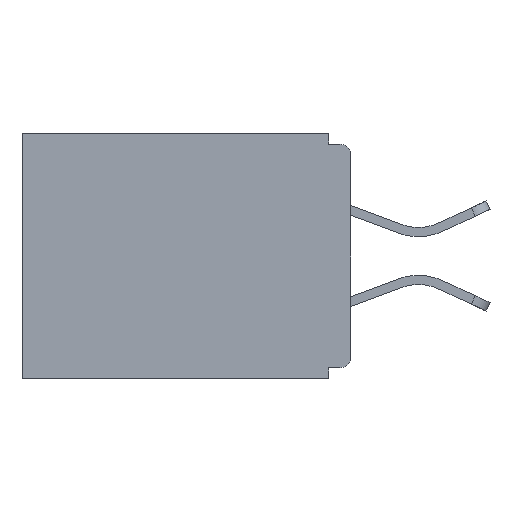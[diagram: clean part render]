
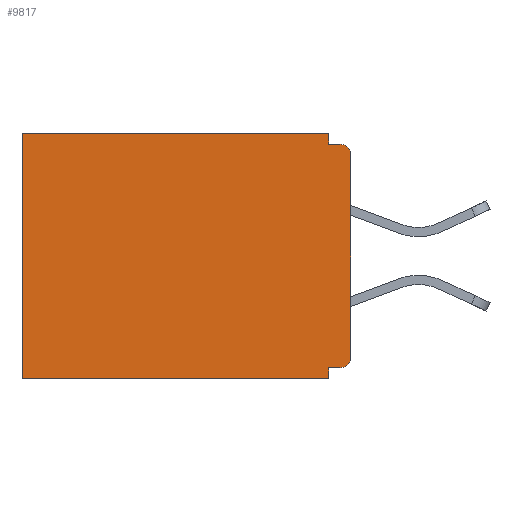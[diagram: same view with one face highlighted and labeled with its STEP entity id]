
A CAD part, left-side view. The second image highlights one B-rep face of the part: STEP entity #9817.
In plain terms, the highlighted planar face has unit normal (-1, 0, 0).
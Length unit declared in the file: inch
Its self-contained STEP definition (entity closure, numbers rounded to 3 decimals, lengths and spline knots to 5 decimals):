
#53 = VERTEX_POINT ( 'NONE', #4305 ) ;
#56 = DIRECTION ( 'NONE',  ( 0., 0., -1. ) ) ;
#120 = VECTOR ( 'NONE', #7833, 39.37008 ) ;
#472 = LINE ( 'NONE', #9594, #2384 ) ;
#532 = ORIENTED_EDGE ( 'NONE', *, *, #11973, .T. ) ;
#645 = DIRECTION ( 'NONE',  ( 0., 0., -1. ) ) ;
#818 = ORIENTED_EDGE ( 'NONE', *, *, #10296, .F. ) ;
#843 = EDGE_CURVE ( 'NONE', #11170, #13612, #1745, .T. ) ;
#1745 = LINE ( 'NONE', #5186, #12698 ) ;
#2384 = VECTOR ( 'NONE', #6439, 39.37008 ) ;
#2605 = DIRECTION ( 'NONE',  ( 0., 0., -1. ) ) ;
#2826 = CARTESIAN_POINT ( 'NONE',  ( 0.298, 0., -0.015 ) ) ;
#2828 = CARTESIAN_POINT ( 'NONE',  ( 0.298, 0.46, 0. ) ) ;
#2873 = DIRECTION ( 'NONE',  ( 0., -1., 0. ) ) ;
#2877 = LINE ( 'NONE', #7743, #120 ) ;
#2940 = LINE ( 'NONE', #10878, #8274 ) ;
#3093 = CARTESIAN_POINT ( 'NONE',  ( 0.298, 0., 0. ) ) ;
#3096 = EDGE_CURVE ( 'NONE', #9137, #13612, #11832, .T. ) ;
#3259 = DIRECTION ( 'NONE',  ( 0., 1., 0. ) ) ;
#3328 = DIRECTION ( 'NONE',  ( 0., 0., -1. ) ) ;
#3933 = LINE ( 'NONE', #2826, #5913 ) ;
#4124 = EDGE_CURVE ( 'NONE', #4360, #11170, #4340, .T. ) ;
#4277 = VERTEX_POINT ( 'NONE', #7335 ) ;
#4305 = CARTESIAN_POINT ( 'NONE',  ( 0.298, 0.015, -0.328 ) ) ;
#4340 = LINE ( 'NONE', #5867, #11533 ) ;
#4360 = VERTEX_POINT ( 'NONE', #8013 ) ;
#4390 = DIRECTION ( 'NONE',  ( 0., 0., -1. ) ) ;
#4479 = VECTOR ( 'NONE', #4390, 39.37008 ) ;
#4544 = CARTESIAN_POINT ( 'NONE',  ( 0.298, 0.031, 0. ) ) ;
#4630 = DIRECTION ( 'NONE',  ( -1., 0., 0. ) ) ;
#4906 = ORIENTED_EDGE ( 'NONE', *, *, #8773, .T. ) ;
#5059 = VERTEX_POINT ( 'NONE', #4544 ) ;
#5186 = CARTESIAN_POINT ( 'NONE',  ( 0.298, 0., -0.343 ) ) ;
#5240 = CARTESIAN_POINT ( 'NONE',  ( 0.298, 0.46, -0.343 ) ) ;
#5397 = ORIENTED_EDGE ( 'NONE', *, *, #10454, .T. ) ;
#5398 = DIRECTION ( 'NONE',  ( 1., 0., 0. ) ) ;
#5611 = EDGE_CURVE ( 'NONE', #11271, #8356, #2940, .T. ) ;
#5690 = CIRCLE ( 'NONE', #11031, 0.015 ) ;
#5867 = CARTESIAN_POINT ( 'NONE',  ( 0.298, 0.031, -0.343 ) ) ;
#5870 = DIRECTION ( 'NONE',  ( -1., 0., 0. ) ) ;
#5886 = ORIENTED_EDGE ( 'NONE', *, *, #12929, .F. ) ;
#5913 = VECTOR ( 'NONE', #2873, 39.37008 ) ;
#6171 = AXIS2_PLACEMENT_3D ( 'NONE', #3093, #5398, #56 ) ;
#6225 = CARTESIAN_POINT ( 'NONE',  ( 0.298, 0., -0.313 ) ) ;
#6432 = ORIENTED_EDGE ( 'NONE', *, *, #843, .F. ) ;
#6437 = CARTESIAN_POINT ( 'NONE',  ( 0.298, 0., -0.328 ) ) ;
#6439 = DIRECTION ( 'NONE',  ( 0., 1., 0. ) ) ;
#6514 = CARTESIAN_POINT ( 'NONE',  ( 0.298, 0.46, 0. ) ) ;
#6520 = ORIENTED_EDGE ( 'NONE', *, *, #4124, .F. ) ;
#6580 = DIRECTION ( 'NONE',  ( 0., 0., -1. ) ) ;
#7241 = DIRECTION ( 'NONE',  ( 0., 1., 0. ) ) ;
#7335 = CARTESIAN_POINT ( 'NONE',  ( 0.298, 0.015, -0.015 ) ) ;
#7743 = CARTESIAN_POINT ( 'NONE',  ( 0.298, 0.031, -0.343 ) ) ;
#7833 = DIRECTION ( 'NONE',  ( 0., 0., -1. ) ) ;
#8013 = CARTESIAN_POINT ( 'NONE',  ( 0.298, 0.031, -0.328 ) ) ;
#8274 = VECTOR ( 'NONE', #3328, 39.37008 ) ;
#8356 = VERTEX_POINT ( 'NONE', #6225 ) ;
#8773 = EDGE_CURVE ( 'NONE', #11271, #4277, #10392, .T. ) ;
#9004 = CARTESIAN_POINT ( 'NONE',  ( 0.298, 0.015, -0.313 ) ) ;
#9137 = VERTEX_POINT ( 'NONE', #2828 ) ;
#9594 = CARTESIAN_POINT ( 'NONE',  ( 0.298, 0., 0. ) ) ;
#9817 = ADVANCED_FACE ( 'NONE', ( #11329 ), #11535, .F. ) ;
#10296 = EDGE_CURVE ( 'NONE', #11020, #4277, #3933, .T. ) ;
#10392 = CIRCLE ( 'NONE', #13238, 0.015 ) ;
#10454 = EDGE_CURVE ( 'NONE', #5059, #9137, #472, .T. ) ;
#10773 = ORIENTED_EDGE ( 'NONE', *, *, #5611, .F. ) ;
#10878 = CARTESIAN_POINT ( 'NONE',  ( 0.298, 0., 0. ) ) ;
#11012 = ORIENTED_EDGE ( 'NONE', *, *, #3096, .T. ) ;
#11020 = VERTEX_POINT ( 'NONE', #11282 ) ;
#11021 = CARTESIAN_POINT ( 'NONE',  ( 0.298, 0., -0.03 ) ) ;
#11031 = AXIS2_PLACEMENT_3D ( 'NONE', #9004, #5870, #2605 ) ;
#11170 = VERTEX_POINT ( 'NONE', #13374 ) ;
#11271 = VERTEX_POINT ( 'NONE', #11021 ) ;
#11282 = CARTESIAN_POINT ( 'NONE',  ( 0.298, 0.031, -0.015 ) ) ;
#11329 = FACE_OUTER_BOUND ( 'NONE', #13463, .T. ) ;
#11533 = VECTOR ( 'NONE', #645, 39.37008 ) ;
#11535 = PLANE ( 'NONE',  #6171 ) ;
#11832 = LINE ( 'NONE', #6514, #4479 ) ;
#11973 = EDGE_CURVE ( 'NONE', #53, #8356, #5690, .T. ) ;
#11996 = CARTESIAN_POINT ( 'NONE',  ( 0.298, 0.015, -0.03 ) ) ;
#12203 = EDGE_CURVE ( 'NONE', #5059, #11020, #2877, .T. ) ;
#12335 = LINE ( 'NONE', #6437, #12674 ) ;
#12674 = VECTOR ( 'NONE', #3259, 39.37008 ) ;
#12698 = VECTOR ( 'NONE', #7241, 39.37008 ) ;
#12929 = EDGE_CURVE ( 'NONE', #53, #4360, #12335, .T. ) ;
#13238 = AXIS2_PLACEMENT_3D ( 'NONE', #11996, #4630, #6580 ) ;
#13275 = ORIENTED_EDGE ( 'NONE', *, *, #12203, .F. ) ;
#13374 = CARTESIAN_POINT ( 'NONE',  ( 0.298, 0.031, -0.343 ) ) ;
#13463 = EDGE_LOOP ( 'NONE', ( #4906, #818, #13275, #5397, #11012, #6432, #6520, #5886, #532, #10773 ) ) ;
#13612 = VERTEX_POINT ( 'NONE', #5240 ) ;
